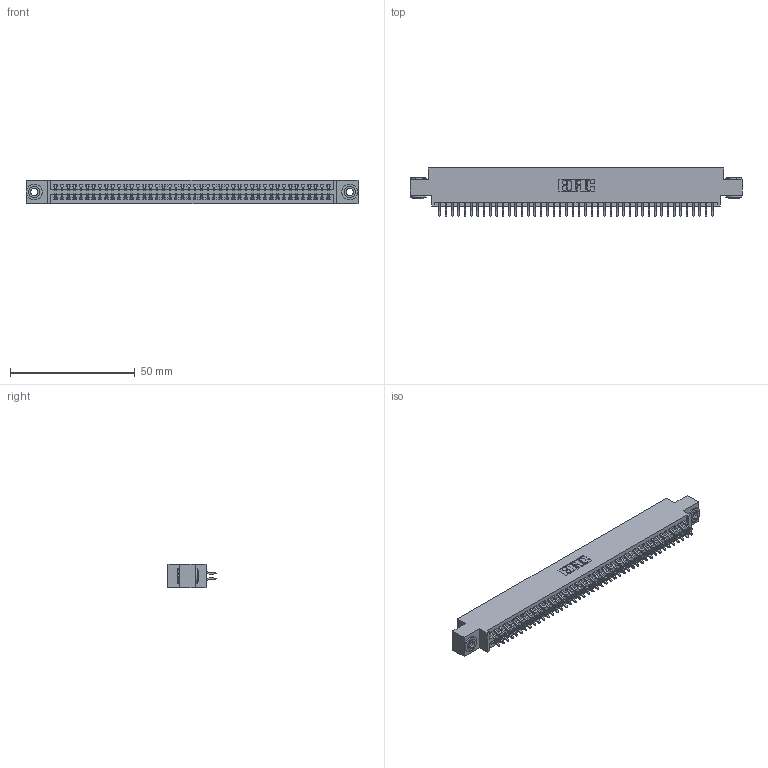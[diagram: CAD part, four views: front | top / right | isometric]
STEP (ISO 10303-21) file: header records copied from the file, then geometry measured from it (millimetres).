
FILE_DESCRIPTION (( 'STEP AP203' ), '1' );
FILE_NAME ('395-088-556-803.STEP', '2019-10-25T14:58:22', ( '' ), ( '' ), 'SwSTEP 2.0', 'SolidWorks 2016', '' );
FILE_SCHEMA (( 'CONFIG_CONTROL_DESIGN' ));
Length unit declared in the file: inch
Products named in the file (4): 345 Part_0.170 Offset - 0.156 Dia-TH; 345-292-001_556 Tail; 345-250-002_345-250-002-102; 395-088-556-803
Assembly tree (91 placements, depth 2):
  395-088-556-803
    345 Part_0.170 Offset - 0.156 Dia-TH
    345-292-001_556 Tail  x88
    345-250-002_345-250-002-102  x2
Bounding box: 132.97 x 19.24 x 9.4 mm (x, y, z)
Volume: 12837.8 mm3; surface area: 19286.5 mm2
Topology: 91 solids, 91 shells, 5096 faces, 15125 edges, 9962 vertices
Faces by surface type: plane 3350, cylinder 1738, cone 8
Entity records: 35256 total; most frequent: CARTESIAN_POINT 5899, ORIENTED_EDGE 5814, DIRECTION 5217, EDGE_CURVE 2907, LINE 2567, VECTOR 2567, VERTEX_POINT 1934, AXIS2_PLACEMENT_3D 1325
